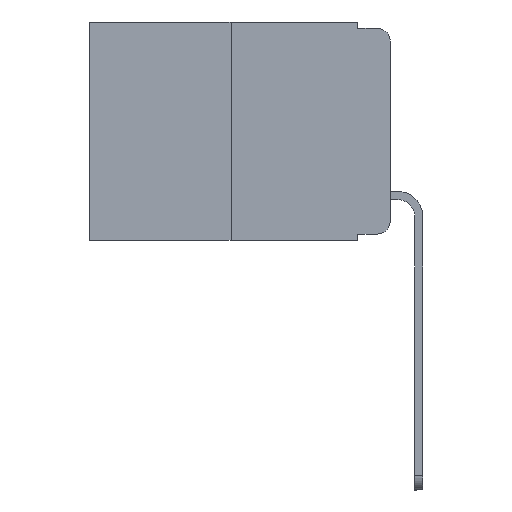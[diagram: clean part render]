
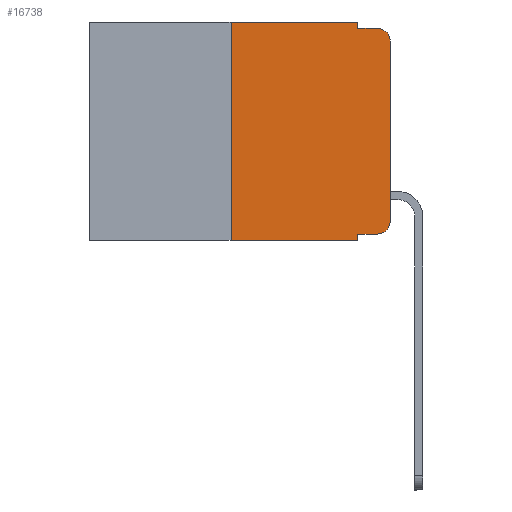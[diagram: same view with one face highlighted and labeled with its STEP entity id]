
A CAD part, left-side view. The second image highlights one B-rep face of the part: STEP entity #16738.
In plain terms, the highlighted planar face has unit normal (-1, 0, 0).
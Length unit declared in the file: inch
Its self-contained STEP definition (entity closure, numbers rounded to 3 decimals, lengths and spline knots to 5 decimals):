
#29 = VERTEX_POINT ( 'NONE', #19888 ) ;
#342 = ORIENTED_EDGE ( 'NONE', *, *, #4075, .T. ) ;
#464 = CARTESIAN_POINT ( 'NONE',  ( 0., 0.02, -0.313 ) ) ;
#666 = DIRECTION ( 'NONE',  ( 0., 0., 1. ) ) ;
#1077 = ORIENTED_EDGE ( 'NONE', *, *, #19250, .T. ) ;
#1684 = AXIS2_PLACEMENT_3D ( 'NONE', #8979, #21932, #10880 ) ;
#1760 = EDGE_CURVE ( 'NONE', #21153, #16262, #21783, .T. ) ;
#1989 = ORIENTED_EDGE ( 'NONE', *, *, #10096, .F. ) ;
#2067 = VERTEX_POINT ( 'NONE', #10450 ) ;
#2283 = VECTOR ( 'NONE', #20499, 39.37008 ) ;
#2400 = DIRECTION ( 'NONE',  ( 0., 0., -1. ) ) ;
#2722 = ORIENTED_EDGE ( 'NONE', *, *, #13900, .F. ) ;
#2960 = CARTESIAN_POINT ( 'NONE',  ( 0., 0.051, -0.01 ) ) ;
#3055 = ORIENTED_EDGE ( 'NONE', *, *, #11701, .T. ) ;
#3111 = CARTESIAN_POINT ( 'NONE',  ( 0., 0.02, -0.333 ) ) ;
#3381 = ORIENTED_EDGE ( 'NONE', *, *, #5733, .F. ) ;
#3390 = VERTEX_POINT ( 'NONE', #22487 ) ;
#4005 = VECTOR ( 'NONE', #10891, 39.37008 ) ;
#4031 = VECTOR ( 'NONE', #666, 39.37008 ) ;
#4075 = EDGE_CURVE ( 'NONE', #24256, #2067, #17727, .T. ) ;
#4092 = CARTESIAN_POINT ( 'NONE',  ( 0., 0., -0.313 ) ) ;
#4505 = CIRCLE ( 'NONE', #1684, 0.02 ) ;
#4785 = FACE_OUTER_BOUND ( 'NONE', #15449, .T. ) ;
#4853 = CARTESIAN_POINT ( 'NONE',  ( 0., 0., 0. ) ) ;
#4985 = EDGE_CURVE ( 'NONE', #21153, #29, #23605, .T. ) ;
#5215 = ORIENTED_EDGE ( 'NONE', *, *, #4985, .T. ) ;
#5238 = VECTOR ( 'NONE', #21321, 39.37008 ) ;
#5733 = EDGE_CURVE ( 'NONE', #3390, #29, #11806, .T. ) ;
#6119 = CARTESIAN_POINT ( 'NONE',  ( 0., 0.25, 0. ) ) ;
#6525 = CARTESIAN_POINT ( 'NONE',  ( 0., 0.473, 0. ) ) ;
#6852 = ORIENTED_EDGE ( 'NONE', *, *, #1760, .F. ) ;
#7375 = CARTESIAN_POINT ( 'NONE',  ( 0., 0.473, 0. ) ) ;
#7582 = VECTOR ( 'NONE', #17876, 39.37008 ) ;
#8089 = VECTOR ( 'NONE', #21382, 39.37008 ) ;
#8191 = LINE ( 'NONE', #6525, #7582 ) ;
#8575 = CARTESIAN_POINT ( 'NONE',  ( 0., 0.473, -0.343 ) ) ;
#8979 = CARTESIAN_POINT ( 'NONE',  ( 0., 0.02, -0.03 ) ) ;
#9037 = ORIENTED_EDGE ( 'NONE', *, *, #19120, .F. ) ;
#9302 = DIRECTION ( 'NONE',  ( 0., 0., -1. ) ) ;
#9993 = AXIS2_PLACEMENT_3D ( 'NONE', #7375, #20428, #9302 ) ;
#10096 = EDGE_CURVE ( 'NONE', #12535, #16119, #15391, .T. ) ;
#10450 = CARTESIAN_POINT ( 'NONE',  ( 0., 0., -0.03 ) ) ;
#10880 = DIRECTION ( 'NONE',  ( 0., 0., -1. ) ) ;
#10891 = DIRECTION ( 'NONE',  ( 0., -1., 0. ) ) ;
#11701 = EDGE_CURVE ( 'NONE', #13494, #24256, #17017, .T. ) ;
#11806 = LINE ( 'NONE', #22560, #21610 ) ;
#12501 = VERTEX_POINT ( 'NONE', #18015 ) ;
#12535 = VERTEX_POINT ( 'NONE', #2960 ) ;
#13160 = LINE ( 'NONE', #19552, #8089 ) ;
#13494 = VERTEX_POINT ( 'NONE', #3111 ) ;
#13900 = EDGE_CURVE ( 'NONE', #12501, #12535, #15393, .T. ) ;
#13967 = DIRECTION ( 'NONE',  ( -1., 0., 0. ) ) ;
#15097 = VECTOR ( 'NONE', #22402, 39.37008 ) ;
#15391 = LINE ( 'NONE', #16449, #4005 ) ;
#15393 = LINE ( 'NONE', #19479, #5238 ) ;
#15449 = EDGE_LOOP ( 'NONE', ( #342, #1077, #1989, #2722, #9037, #6852, #5215, #3381, #16487, #3055 ) ) ;
#16119 = VERTEX_POINT ( 'NONE', #22190 ) ;
#16262 = VERTEX_POINT ( 'NONE', #18918 ) ;
#16449 = CARTESIAN_POINT ( 'NONE',  ( 0., 0.051, -0.01 ) ) ;
#16487 = ORIENTED_EDGE ( 'NONE', *, *, #20812, .T. ) ;
#16738 = ADVANCED_FACE ( 'NONE', ( #4785 ), #18568, .F. ) ;
#17017 = CIRCLE ( 'NONE', #20462, 0.02 ) ;
#17727 = LINE ( 'NONE', #4853, #4031 ) ;
#17876 = DIRECTION ( 'NONE',  ( 0., -1., 0. ) ) ;
#18015 = CARTESIAN_POINT ( 'NONE',  ( 0., 0.051, 0. ) ) ;
#18568 = PLANE ( 'NONE',  #9993 ) ;
#18918 = CARTESIAN_POINT ( 'NONE',  ( 0., 0.25, 0. ) ) ;
#19120 = EDGE_CURVE ( 'NONE', #16262, #12501, #8191, .T. ) ;
#19250 = EDGE_CURVE ( 'NONE', #2067, #16119, #4505, .T. ) ;
#19479 = CARTESIAN_POINT ( 'NONE',  ( 0., 0.051, 0. ) ) ;
#19552 = CARTESIAN_POINT ( 'NONE',  ( 0., 0.051, -0.333 ) ) ;
#19888 = CARTESIAN_POINT ( 'NONE',  ( 0., 0.051, -0.343 ) ) ;
#20428 = DIRECTION ( 'NONE',  ( 1., 0., 0. ) ) ;
#20462 = AXIS2_PLACEMENT_3D ( 'NONE', #464, #13967, #2400 ) ;
#20499 = DIRECTION ( 'NONE',  ( 0., 0., 1. ) ) ;
#20812 = EDGE_CURVE ( 'NONE', #3390, #13494, #13160, .T. ) ;
#21153 = VERTEX_POINT ( 'NONE', #21987 ) ;
#21321 = DIRECTION ( 'NONE',  ( 0., 0., -1. ) ) ;
#21382 = DIRECTION ( 'NONE',  ( 0., -1., 0. ) ) ;
#21545 = DIRECTION ( 'NONE',  ( 0., 0., -1. ) ) ;
#21610 = VECTOR ( 'NONE', #21545, 39.37008 ) ;
#21783 = LINE ( 'NONE', #6119, #2283 ) ;
#21932 = DIRECTION ( 'NONE',  ( -1., 0., 0. ) ) ;
#21987 = CARTESIAN_POINT ( 'NONE',  ( 0., 0.25, -0.343 ) ) ;
#22190 = CARTESIAN_POINT ( 'NONE',  ( 0., 0.02, -0.01 ) ) ;
#22402 = DIRECTION ( 'NONE',  ( 0., -1., 0. ) ) ;
#22487 = CARTESIAN_POINT ( 'NONE',  ( 0., 0.051, -0.333 ) ) ;
#22560 = CARTESIAN_POINT ( 'NONE',  ( 0., 0.051, 0. ) ) ;
#23605 = LINE ( 'NONE', #8575, #15097 ) ;
#24256 = VERTEX_POINT ( 'NONE', #4092 ) ;
